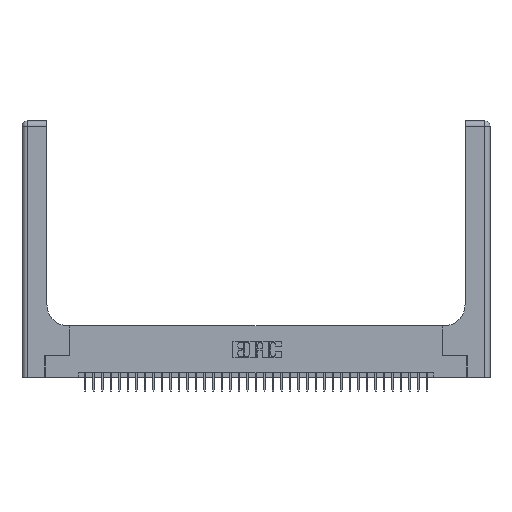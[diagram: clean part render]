
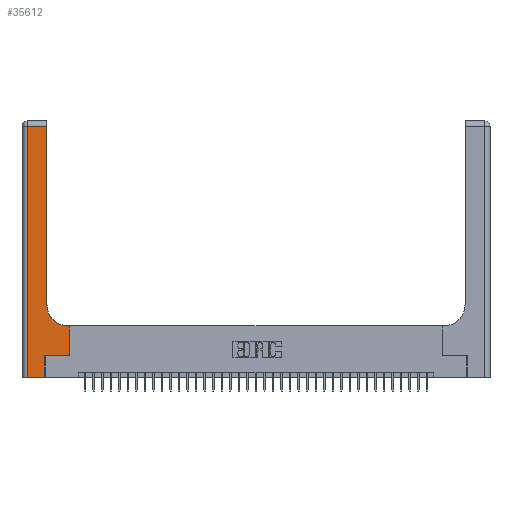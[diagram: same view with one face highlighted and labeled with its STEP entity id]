
A CAD part, top view. The second image highlights one B-rep face of the part: STEP entity #35612.
In plain terms, the highlighted planar face has unit normal (0, 0, 1).
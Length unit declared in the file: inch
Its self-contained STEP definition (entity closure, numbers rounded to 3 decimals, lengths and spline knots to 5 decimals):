
#244 = VECTOR ( 'NONE', #25775, 39.37008 ) ;
#337 = DIRECTION ( 'NONE',  ( -1., 0., 0. ) ) ;
#1335 = CARTESIAN_POINT ( 'NONE',  ( 0.2915, 3., 0.37 ) ) ;
#2323 = CARTESIAN_POINT ( 'NONE',  ( 0.5585, 0.25, 0.37 ) ) ;
#2769 = EDGE_CURVE ( 'NONE', #20280, #5113, #15970, .T. ) ;
#3096 = DIRECTION ( 'NONE',  ( 0., 1., 0. ) ) ;
#3106 = LINE ( 'NONE', #13038, #32134 ) ;
#3801 = DIRECTION ( 'NONE',  ( -1., 0., 0. ) ) ;
#4060 = VERTEX_POINT ( 'NONE', #25471 ) ;
#4132 = EDGE_CURVE ( 'NONE', #12629, #21922, #26207, .T. ) ;
#4561 = CARTESIAN_POINT ( 'NONE',  ( 0.2915, 0.85, 0.37 ) ) ;
#4747 = ORIENTED_EDGE ( 'NONE', *, *, #35424, .T. ) ;
#5113 = VERTEX_POINT ( 'NONE', #25397 ) ;
#5332 = EDGE_CURVE ( 'NONE', #22734, #4060, #27461, .T. ) ;
#5554 = CARTESIAN_POINT ( 'NONE',  ( 0.06, 2.94, 0.37 ) ) ;
#5777 = ORIENTED_EDGE ( 'NONE', *, *, #16552, .T. ) ;
#6006 = LINE ( 'NONE', #6821, #20606 ) ;
#6620 = DIRECTION ( 'NONE',  ( 0., 0., -1. ) ) ;
#6821 = CARTESIAN_POINT ( 'NONE',  ( 0., 2.94, 0.37 ) ) ;
#7251 = CIRCLE ( 'NONE', #11645, 0.25 ) ;
#7354 = DIRECTION ( 'NONE',  ( 0., 1., 0. ) ) ;
#7803 = LINE ( 'NONE', #1335, #37495 ) ;
#8034 = EDGE_CURVE ( 'NONE', #16379, #20280, #6006, .T. ) ;
#8404 = CARTESIAN_POINT ( 'NONE',  ( 0.269, 0., 0.37 ) ) ;
#9004 = FACE_OUTER_BOUND ( 'NONE', #16617, .T. ) ;
#9219 = ORIENTED_EDGE ( 'NONE', *, *, #26897, .T. ) ;
#9321 = ORIENTED_EDGE ( 'NONE', *, *, #4132, .T. ) ;
#9655 = AXIS2_PLACEMENT_3D ( 'NONE', #15064, #17992, #337 ) ;
#10545 = ORIENTED_EDGE ( 'NONE', *, *, #21901, .T. ) ;
#11645 = AXIS2_PLACEMENT_3D ( 'NONE', #24007, #6620, #26876 ) ;
#12145 = PLANE ( 'NONE',  #9655 ) ;
#12369 = CARTESIAN_POINT ( 'NONE',  ( 0.2915, 2.94, 0.37 ) ) ;
#12629 = VERTEX_POINT ( 'NONE', #22919 ) ;
#13038 = CARTESIAN_POINT ( 'NONE',  ( 0., 0., 0.37 ) ) ;
#13247 = DIRECTION ( 'NONE',  ( -1., 0., 0. ) ) ;
#14025 = VERTEX_POINT ( 'NONE', #31568 ) ;
#14981 = EDGE_CURVE ( 'NONE', #5113, #12629, #3106, .T. ) ;
#15064 = CARTESIAN_POINT ( 'NONE',  ( 0., 3., 0.37 ) ) ;
#15970 = LINE ( 'NONE', #22892, #244 ) ;
#15990 = DIRECTION ( 'NONE',  ( 1., 0., 0. ) ) ;
#16089 = CARTESIAN_POINT ( 'NONE',  ( 0.2915, 0.6, 0.37 ) ) ;
#16165 = CARTESIAN_POINT ( 'NONE',  ( 0.269, 0.25, 0.37 ) ) ;
#16379 = VERTEX_POINT ( 'NONE', #12369 ) ;
#16552 = EDGE_CURVE ( 'NONE', #4060, #14025, #19544, .T. ) ;
#16617 = EDGE_LOOP ( 'NONE', ( #10545, #18737, #33513, #24247, #9321, #4747, #35945, #5777, #9219 ) ) ;
#17126 = DIRECTION ( 'NONE',  ( 1., 0., 0. ) ) ;
#17734 = CARTESIAN_POINT ( 'NONE',  ( 0.5585, 0.25, 0.37 ) ) ;
#17992 = DIRECTION ( 'NONE',  ( 0., 0., -1. ) ) ;
#18575 = VECTOR ( 'NONE', #34295, 39.37008 ) ;
#18737 = ORIENTED_EDGE ( 'NONE', *, *, #8034, .T. ) ;
#18953 = VECTOR ( 'NONE', #3096, 39.37008 ) ;
#19395 = VERTEX_POINT ( 'NONE', #4561 ) ;
#19544 = LINE ( 'NONE', #16089, #27154 ) ;
#20280 = VERTEX_POINT ( 'NONE', #5554 ) ;
#20606 = VECTOR ( 'NONE', #3801, 39.37008 ) ;
#21901 = EDGE_CURVE ( 'NONE', #19395, #16379, #7803, .T. ) ;
#21922 = VERTEX_POINT ( 'NONE', #16165 ) ;
#22734 = VERTEX_POINT ( 'NONE', #2323 ) ;
#22892 = CARTESIAN_POINT ( 'NONE',  ( 0.06, 3., 0.37 ) ) ;
#22919 = CARTESIAN_POINT ( 'NONE',  ( 0.269, 0., 0.37 ) ) ;
#24007 = CARTESIAN_POINT ( 'NONE',  ( 0.5415, 0.85, 0.37 ) ) ;
#24247 = ORIENTED_EDGE ( 'NONE', *, *, #14981, .T. ) ;
#25397 = CARTESIAN_POINT ( 'NONE',  ( 0.06, 0., 0.37 ) ) ;
#25471 = CARTESIAN_POINT ( 'NONE',  ( 0.5585, 0.6, 0.37 ) ) ;
#25775 = DIRECTION ( 'NONE',  ( 0., -1., 0. ) ) ;
#26207 = LINE ( 'NONE', #8404, #18575 ) ;
#26876 = DIRECTION ( 'NONE',  ( 1., 0., 0. ) ) ;
#26897 = EDGE_CURVE ( 'NONE', #14025, #19395, #7251, .T. ) ;
#27154 = VECTOR ( 'NONE', #13247, 39.37008 ) ;
#27461 = LINE ( 'NONE', #17734, #18953 ) ;
#28868 = VECTOR ( 'NONE', #17126, 39.37008 ) ;
#29750 = LINE ( 'NONE', #31399, #28868 ) ;
#31399 = CARTESIAN_POINT ( 'NONE',  ( 0.269, 0.25, 0.37 ) ) ;
#31568 = CARTESIAN_POINT ( 'NONE',  ( 0.5415, 0.6, 0.37 ) ) ;
#32134 = VECTOR ( 'NONE', #15990, 39.37008 ) ;
#33513 = ORIENTED_EDGE ( 'NONE', *, *, #2769, .T. ) ;
#34295 = DIRECTION ( 'NONE',  ( 0., 1., 0. ) ) ;
#35424 = EDGE_CURVE ( 'NONE', #21922, #22734, #29750, .T. ) ;
#35612 = ADVANCED_FACE ( 'NONE', ( #9004 ), #12145, .F. ) ;
#35945 = ORIENTED_EDGE ( 'NONE', *, *, #5332, .T. ) ;
#37495 = VECTOR ( 'NONE', #7354, 39.37008 ) ;
